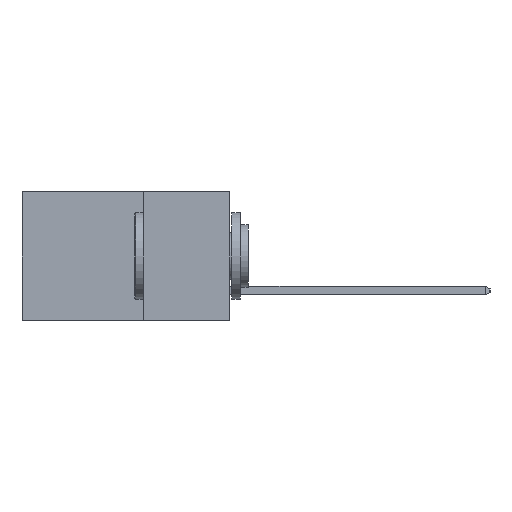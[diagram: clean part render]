
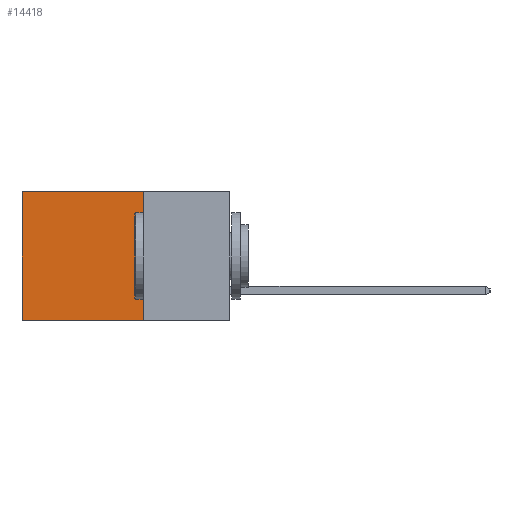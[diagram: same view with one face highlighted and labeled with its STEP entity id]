
A CAD part, left-side view. The second image highlights one B-rep face of the part: STEP entity #14418.
In plain terms, the highlighted planar face has unit normal (-1, 0, 0).
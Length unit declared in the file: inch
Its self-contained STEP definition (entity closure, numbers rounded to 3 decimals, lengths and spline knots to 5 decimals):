
#30 = CARTESIAN_POINT ( 'NONE',  ( 0.2615, 0.25, 0. ) ) ;
#346 = AXIS2_PLACEMENT_3D ( 'NONE', #11708, #13507, #2662 ) ;
#619 = VECTOR ( 'NONE', #1782, 39.37008 ) ;
#1185 = CARTESIAN_POINT ( 'NONE',  ( 0.2615, 0.25, -0.37 ) ) ;
#1779 = VECTOR ( 'NONE', #11855, 39.37008 ) ;
#1782 = DIRECTION ( 'NONE',  ( 0., 0., -1. ) ) ;
#2341 = CARTESIAN_POINT ( 'NONE',  ( 0.2615, 0.6, -0.37 ) ) ;
#2361 = LINE ( 'NONE', #11950, #1779 ) ;
#2662 = DIRECTION ( 'NONE',  ( 0., 0., -1. ) ) ;
#3406 = CARTESIAN_POINT ( 'NONE',  ( 0.2615, 0.6, 0. ) ) ;
#4941 = ORIENTED_EDGE ( 'NONE', *, *, #7000, .F. ) ;
#6287 = VERTEX_POINT ( 'NONE', #3406 ) ;
#6518 = VERTEX_POINT ( 'NONE', #17128 ) ;
#6630 = LINE ( 'NONE', #1185, #20052 ) ;
#7000 = EDGE_CURVE ( 'NONE', #18349, #6518, #6630, .T. ) ;
#7176 = VERTEX_POINT ( 'NONE', #30 ) ;
#7250 = EDGE_CURVE ( 'NONE', #7176, #6287, #19257, .T. ) ;
#9646 = DIRECTION ( 'NONE',  ( 0., 1., 0. ) ) ;
#10003 = VECTOR ( 'NONE', #19197, 39.37008 ) ;
#10487 = EDGE_CURVE ( 'NONE', #7176, #18349, #2361, .T. ) ;
#11171 = FACE_OUTER_BOUND ( 'NONE', #13007, .T. ) ;
#11310 = CARTESIAN_POINT ( 'NONE',  ( 0.2615, 0.25, -0.37 ) ) ;
#11332 = ORIENTED_EDGE ( 'NONE', *, *, #11475, .T. ) ;
#11475 = EDGE_CURVE ( 'NONE', #6287, #6518, #15516, .T. ) ;
#11708 = CARTESIAN_POINT ( 'NONE',  ( 0.2615, 0.25, -0.37 ) ) ;
#11855 = DIRECTION ( 'NONE',  ( 0., 0., -1. ) ) ;
#11950 = CARTESIAN_POINT ( 'NONE',  ( 0.2615, 0.25, -0.37 ) ) ;
#13007 = EDGE_LOOP ( 'NONE', ( #11332, #4941, #16994, #17695 ) ) ;
#13507 = DIRECTION ( 'NONE',  ( 1., 0., 0. ) ) ;
#14418 = ADVANCED_FACE ( 'NONE', ( #11171 ), #21974, .F. ) ;
#15516 = LINE ( 'NONE', #2341, #619 ) ;
#16994 = ORIENTED_EDGE ( 'NONE', *, *, #10487, .F. ) ;
#17128 = CARTESIAN_POINT ( 'NONE',  ( 0.2615, 0.6, -0.37 ) ) ;
#17695 = ORIENTED_EDGE ( 'NONE', *, *, #7250, .T. ) ;
#18349 = VERTEX_POINT ( 'NONE', #11310 ) ;
#19197 = DIRECTION ( 'NONE',  ( 0., 1., 0. ) ) ;
#19257 = LINE ( 'NONE', #20082, #10003 ) ;
#20052 = VECTOR ( 'NONE', #9646, 39.37008 ) ;
#20082 = CARTESIAN_POINT ( 'NONE',  ( 0.2615, 0.25, 0. ) ) ;
#21974 = PLANE ( 'NONE',  #346 ) ;
